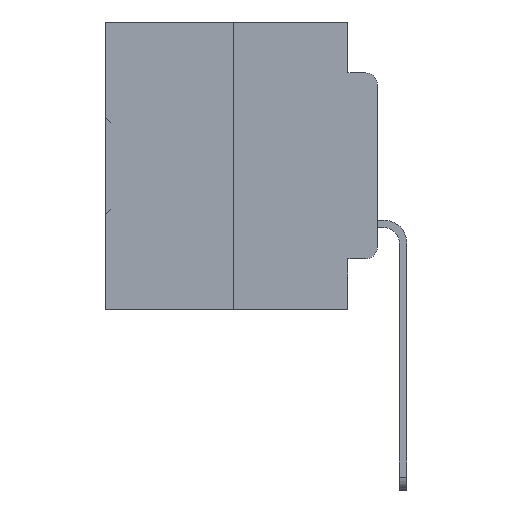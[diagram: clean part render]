
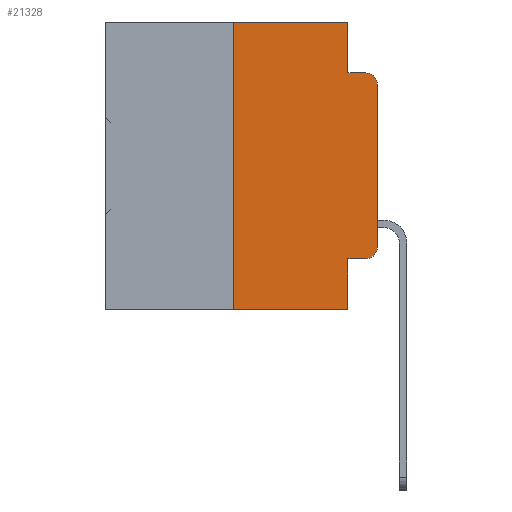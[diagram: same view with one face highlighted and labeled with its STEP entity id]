
A CAD part, left-side view. The second image highlights one B-rep face of the part: STEP entity #21328.
In plain terms, the highlighted planar face has unit normal (-1, 0, 0).
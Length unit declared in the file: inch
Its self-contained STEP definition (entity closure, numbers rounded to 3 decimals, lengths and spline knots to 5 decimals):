
#478 = CARTESIAN_POINT ( 'NONE',  ( 0., 0.02, -0.4115 ) ) ;
#708 = LINE ( 'NONE', #30830, #31275 ) ;
#857 = CARTESIAN_POINT ( 'NONE',  ( 0., 0., -0.1085 ) ) ;
#891 = ORIENTED_EDGE ( 'NONE', *, *, #11949, .T. ) ;
#1321 = LINE ( 'NONE', #33444, #9243 ) ;
#1534 = CARTESIAN_POINT ( 'NONE',  ( 0., 0.051, -0.5 ) ) ;
#1598 = VECTOR ( 'NONE', #20826, 39.37008 ) ;
#1776 = VERTEX_POINT ( 'NONE', #14747 ) ;
#2510 = EDGE_CURVE ( 'NONE', #15420, #1776, #32083, .T. ) ;
#2852 = ORIENTED_EDGE ( 'NONE', *, *, #15971, .F. ) ;
#3223 = VECTOR ( 'NONE', #3873, 39.37008 ) ;
#3242 = DIRECTION ( 'NONE',  ( -1., 0., 0. ) ) ;
#3563 = EDGE_CURVE ( 'NONE', #11823, #11142, #15813, .T. ) ;
#3873 = DIRECTION ( 'NONE',  ( 0., 0., -1. ) ) ;
#4103 = CARTESIAN_POINT ( 'NONE',  ( 0., 0.051, 0. ) ) ;
#4308 = EDGE_CURVE ( 'NONE', #35770, #4376, #24644, .T. ) ;
#4321 = CARTESIAN_POINT ( 'NONE',  ( 0., 0.25, -0.5 ) ) ;
#4376 = VERTEX_POINT ( 'NONE', #35174 ) ;
#5730 = ORIENTED_EDGE ( 'NONE', *, *, #36609, .T. ) ;
#5801 = EDGE_CURVE ( 'NONE', #29797, #35770, #21499, .T. ) ;
#6174 = DIRECTION ( 'NONE',  ( 0., 0., 1. ) ) ;
#7116 = AXIS2_PLACEMENT_3D ( 'NONE', #8510, #34018, #17230 ) ;
#7399 = AXIS2_PLACEMENT_3D ( 'NONE', #25850, #8828, #28688 ) ;
#8510 = CARTESIAN_POINT ( 'NONE',  ( 0., 0.473, 0. ) ) ;
#8576 = FACE_OUTER_BOUND ( 'NONE', #31062, .T. ) ;
#8828 = DIRECTION ( 'NONE',  ( -1., 0., 0. ) ) ;
#9203 = VERTEX_POINT ( 'NONE', #21125 ) ;
#9243 = VECTOR ( 'NONE', #16622, 39.37008 ) ;
#9829 = ORIENTED_EDGE ( 'NONE', *, *, #17934, .T. ) ;
#10335 = VERTEX_POINT ( 'NONE', #1534 ) ;
#11068 = LINE ( 'NONE', #29626, #3223 ) ;
#11142 = VERTEX_POINT ( 'NONE', #857 ) ;
#11823 = VERTEX_POINT ( 'NONE', #24607 ) ;
#11949 = EDGE_CURVE ( 'NONE', #15420, #10335, #708, .T. ) ;
#12609 = DIRECTION ( 'NONE',  ( 0., -1., 0. ) ) ;
#12890 = VECTOR ( 'NONE', #12609, 39.37008 ) ;
#13982 = VECTOR ( 'NONE', #18697, 39.37008 ) ;
#14747 = CARTESIAN_POINT ( 'NONE',  ( 0., 0.25, 0. ) ) ;
#15420 = VERTEX_POINT ( 'NONE', #4321 ) ;
#15791 = AXIS2_PLACEMENT_3D ( 'NONE', #20548, #3242, #23387 ) ;
#15813 = LINE ( 'NONE', #23324, #31616 ) ;
#15932 = EDGE_CURVE ( 'NONE', #1776, #29797, #27026, .T. ) ;
#15971 = EDGE_CURVE ( 'NONE', #9203, #10335, #11068, .T. ) ;
#16125 = ORIENTED_EDGE ( 'NONE', *, *, #3563, .T. ) ;
#16221 = CARTESIAN_POINT ( 'NONE',  ( 0., 0.051, -0.0885 ) ) ;
#16622 = DIRECTION ( 'NONE',  ( 0., -1., 0. ) ) ;
#17230 = DIRECTION ( 'NONE',  ( 0., 0., -1. ) ) ;
#17861 = ORIENTED_EDGE ( 'NONE', *, *, #15932, .F. ) ;
#17934 = EDGE_CURVE ( 'NONE', #11142, #4376, #20860, .T. ) ;
#18697 = DIRECTION ( 'NONE',  ( 0., 0., -1. ) ) ;
#19924 = PLANE ( 'NONE',  #7116 ) ;
#20548 = CARTESIAN_POINT ( 'NONE',  ( 0., 0.02, -0.1085 ) ) ;
#20826 = DIRECTION ( 'NONE',  ( 0., -1., 0. ) ) ;
#20860 = CIRCLE ( 'NONE', #15791, 0.02 ) ;
#21125 = CARTESIAN_POINT ( 'NONE',  ( 0., 0.051, -0.4115 ) ) ;
#21328 = ADVANCED_FACE ( 'NONE', ( #8576 ), #19924, .F. ) ;
#21499 = LINE ( 'NONE', #4103, #13982 ) ;
#22612 = CARTESIAN_POINT ( 'NONE',  ( 0., 0.25, 0. ) ) ;
#23324 = CARTESIAN_POINT ( 'NONE',  ( 0., 0., 0. ) ) ;
#23387 = DIRECTION ( 'NONE',  ( 0., 0., -1. ) ) ;
#24423 = EDGE_CURVE ( 'NONE', #9203, #32804, #1321, .T. ) ;
#24607 = CARTESIAN_POINT ( 'NONE',  ( 0., 0., -0.3915 ) ) ;
#24621 = VECTOR ( 'NONE', #31053, 39.37008 ) ;
#24644 = LINE ( 'NONE', #29183, #1598 ) ;
#24858 = ORIENTED_EDGE ( 'NONE', *, *, #5801, .F. ) ;
#25850 = CARTESIAN_POINT ( 'NONE',  ( 0., 0.02, -0.3915 ) ) ;
#26686 = CARTESIAN_POINT ( 'NONE',  ( 0., 0.473, 0. ) ) ;
#27026 = LINE ( 'NONE', #26686, #12890 ) ;
#27149 = ORIENTED_EDGE ( 'NONE', *, *, #24423, .T. ) ;
#28028 = DIRECTION ( 'NONE',  ( 0., -1., 0. ) ) ;
#28688 = DIRECTION ( 'NONE',  ( 0., 0., -1. ) ) ;
#29183 = CARTESIAN_POINT ( 'NONE',  ( 0., 0.051, -0.0885 ) ) ;
#29247 = ORIENTED_EDGE ( 'NONE', *, *, #2510, .F. ) ;
#29626 = CARTESIAN_POINT ( 'NONE',  ( 0., 0.051, 0. ) ) ;
#29797 = VERTEX_POINT ( 'NONE', #30566 ) ;
#29856 = CIRCLE ( 'NONE', #7399, 0.02 ) ;
#30566 = CARTESIAN_POINT ( 'NONE',  ( 0., 0.051, 0. ) ) ;
#30830 = CARTESIAN_POINT ( 'NONE',  ( 0., 0.473, -0.5 ) ) ;
#31053 = DIRECTION ( 'NONE',  ( 0., 0., 1. ) ) ;
#31062 = EDGE_LOOP ( 'NONE', ( #16125, #9829, #35310, #24858, #17861, #29247, #891, #2852, #27149, #5730 ) ) ;
#31275 = VECTOR ( 'NONE', #28028, 39.37008 ) ;
#31616 = VECTOR ( 'NONE', #6174, 39.37008 ) ;
#32083 = LINE ( 'NONE', #22612, #24621 ) ;
#32804 = VERTEX_POINT ( 'NONE', #478 ) ;
#33444 = CARTESIAN_POINT ( 'NONE',  ( 0., 0.051, -0.4115 ) ) ;
#34018 = DIRECTION ( 'NONE',  ( 1., 0., 0. ) ) ;
#35174 = CARTESIAN_POINT ( 'NONE',  ( 0., 0.02, -0.0885 ) ) ;
#35310 = ORIENTED_EDGE ( 'NONE', *, *, #4308, .F. ) ;
#35770 = VERTEX_POINT ( 'NONE', #16221 ) ;
#36609 = EDGE_CURVE ( 'NONE', #32804, #11823, #29856, .T. ) ;
